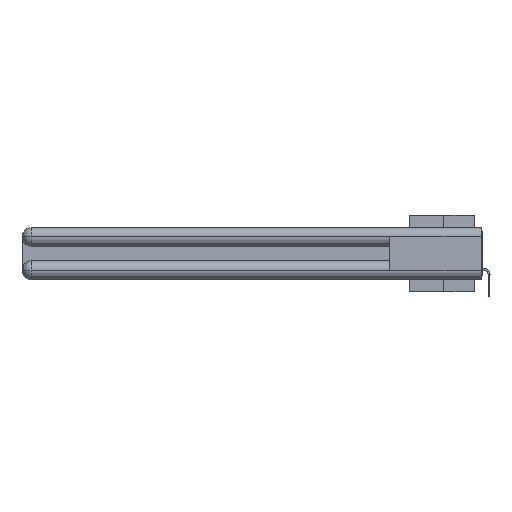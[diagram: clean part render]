
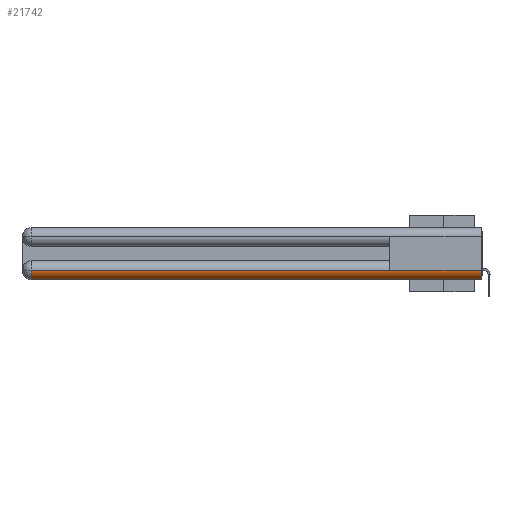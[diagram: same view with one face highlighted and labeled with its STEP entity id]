
A CAD part, left-side view. The second image highlights one B-rep face of the part: STEP entity #21742.
In plain terms, the highlighted cylindrical face has radius 1.562 mm (diameter 3.124 mm), a partial arc.
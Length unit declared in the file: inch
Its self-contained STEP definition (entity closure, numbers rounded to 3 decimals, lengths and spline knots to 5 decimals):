
#2 = VECTOR ( 'NONE', #31062, 39.37008 ) ;
#174 = AXIS2_PLACEMENT_3D ( 'NONE', #31335, #20891, #26018 ) ;
#1074 = EDGE_LOOP ( 'NONE', ( #10484, #10805, #32143, #27832, #29969 ) ) ;
#3437 = EDGE_CURVE ( 'NONE', #31148, #28710, #18074, .T. ) ;
#3726 = AXIS2_PLACEMENT_3D ( 'NONE', #32354, #19730, #25036 ) ;
#3789 = EDGE_CURVE ( 'NONE', #28710, #10071, #27719, .T. ) ;
#4294 = AXIS2_PLACEMENT_3D ( 'NONE', #25921, #22742, #18281 ) ;
#8906 = CARTESIAN_POINT ( 'NONE',  ( 0.0615, 2.94, -0.34 ) ) ;
#9223 = CIRCLE ( 'NONE', #174, 0.0615 ) ;
#10071 = VERTEX_POINT ( 'NONE', #8906 ) ;
#10484 = ORIENTED_EDGE ( 'NONE', *, *, #3437, .T. ) ;
#10805 = ORIENTED_EDGE ( 'NONE', *, *, #3789, .T. ) ;
#13044 = CARTESIAN_POINT ( 'NONE',  ( 0., 0.6, -0.2785 ) ) ;
#15606 = FACE_OUTER_BOUND ( 'NONE', #1074, .T. ) ;
#15648 = VERTEX_POINT ( 'NONE', #20375 ) ;
#16072 = CARTESIAN_POINT ( 'NONE',  ( 0., 0., -0.2785 ) ) ;
#18074 = LINE ( 'NONE', #16072, #2 ) ;
#18243 = EDGE_CURVE ( 'NONE', #32258, #10071, #27174, .T. ) ;
#18281 = DIRECTION ( 'NONE',  ( 0., 0., -1. ) ) ;
#18635 = VECTOR ( 'NONE', #27655, 39.37008 ) ;
#19286 = CARTESIAN_POINT ( 'NONE',  ( 0.0615, 0., -0.34 ) ) ;
#19730 = DIRECTION ( 'NONE',  ( 0., -1., 0. ) ) ;
#20375 = CARTESIAN_POINT ( 'NONE',  ( 0., 0., -0.2785 ) ) ;
#20891 = DIRECTION ( 'NONE',  ( 0., -1., 0. ) ) ;
#21742 = ADVANCED_FACE ( 'NONE', ( #15606 ), #32898, .T. ) ;
#22434 = VECTOR ( 'NONE', #25217, 39.37008 ) ;
#22742 = DIRECTION ( 'NONE',  ( 0., -1., 0. ) ) ;
#24452 = EDGE_CURVE ( 'NONE', #15648, #32258, #9223, .T. ) ;
#25036 = DIRECTION ( 'NONE',  ( 0., 0., 1. ) ) ;
#25217 = DIRECTION ( 'NONE',  ( 0., -1., 0. ) ) ;
#25606 = CARTESIAN_POINT ( 'NONE',  ( 0., 2.94, -0.2785 ) ) ;
#25921 = CARTESIAN_POINT ( 'NONE',  ( 0.0615, 0., -0.2785 ) ) ;
#26018 = DIRECTION ( 'NONE',  ( 1., 0., 0. ) ) ;
#27174 = LINE ( 'NONE', #27347, #18635 ) ;
#27347 = CARTESIAN_POINT ( 'NONE',  ( 0.0615, 0., -0.34 ) ) ;
#27655 = DIRECTION ( 'NONE',  ( 0., 1., 0. ) ) ;
#27719 = CIRCLE ( 'NONE', #3726, 0.0615 ) ;
#27832 = ORIENTED_EDGE ( 'NONE', *, *, #24452, .F. ) ;
#28710 = VERTEX_POINT ( 'NONE', #25606 ) ;
#29872 = LINE ( 'NONE', #30195, #22434 ) ;
#29969 = ORIENTED_EDGE ( 'NONE', *, *, #32826, .F. ) ;
#30195 = CARTESIAN_POINT ( 'NONE',  ( 0., 0., -0.2785 ) ) ;
#31062 = DIRECTION ( 'NONE',  ( 0., 1., 0. ) ) ;
#31148 = VERTEX_POINT ( 'NONE', #13044 ) ;
#31335 = CARTESIAN_POINT ( 'NONE',  ( 0.0615, 0., -0.2785 ) ) ;
#32143 = ORIENTED_EDGE ( 'NONE', *, *, #18243, .F. ) ;
#32258 = VERTEX_POINT ( 'NONE', #19286 ) ;
#32354 = CARTESIAN_POINT ( 'NONE',  ( 0.0615, 2.94, -0.2785 ) ) ;
#32826 = EDGE_CURVE ( 'NONE', #31148, #15648, #29872, .T. ) ;
#32898 = CYLINDRICAL_SURFACE ( 'NONE', #4294, 0.0615 ) ;
